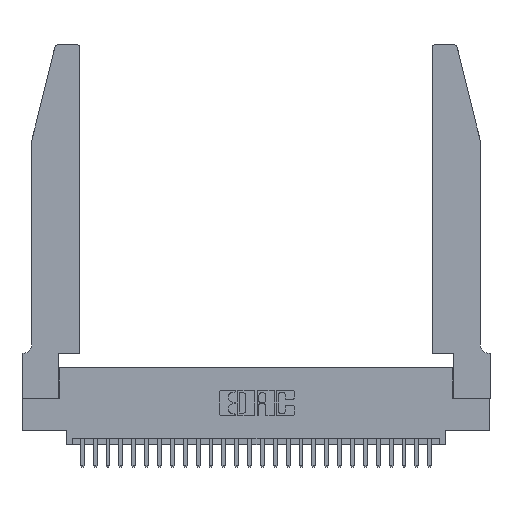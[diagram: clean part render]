
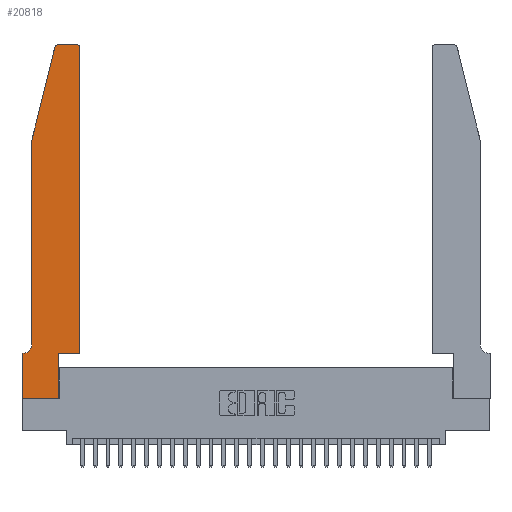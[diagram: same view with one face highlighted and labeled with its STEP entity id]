
A CAD part, top view. The second image highlights one B-rep face of the part: STEP entity #20818.
In plain terms, the highlighted planar face has unit normal (0, 0, 1).
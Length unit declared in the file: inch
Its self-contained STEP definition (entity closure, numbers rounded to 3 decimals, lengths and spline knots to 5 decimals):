
#77 = ORIENTED_EDGE ( 'NONE', *, *, #12620, .T. ) ;
#313 = LINE ( 'NONE', #23612, #17528 ) ;
#765 = VECTOR ( 'NONE', #23305, 39.37008 ) ;
#925 = ORIENTED_EDGE ( 'NONE', *, *, #25373, .T. ) ;
#2102 = ORIENTED_EDGE ( 'NONE', *, *, #21250, .T. ) ;
#2154 = CIRCLE ( 'NONE', #4100, 0.03 ) ;
#2333 = CARTESIAN_POINT ( 'NONE',  ( 0., 0., 0.37 ) ) ;
#2403 = CARTESIAN_POINT ( 'NONE',  ( 0.4505, 0.35, 0.37 ) ) ;
#2539 = LINE ( 'NONE', #8408, #19004 ) ;
#3184 = CARTESIAN_POINT ( 'NONE',  ( 0.0755, 0.35, 0.37 ) ) ;
#3295 = LINE ( 'NONE', #2333, #15235 ) ;
#3737 = LINE ( 'NONE', #22933, #20849 ) ;
#4062 = ORIENTED_EDGE ( 'NONE', *, *, #21682, .T. ) ;
#4100 = AXIS2_PLACEMENT_3D ( 'NONE', #22293, #8950, #24520 ) ;
#5616 = CARTESIAN_POINT ( 'NONE',  ( 0.0755, 2., 0.37 ) ) ;
#5730 = CARTESIAN_POINT ( 'NONE',  ( 0.25487, 2.72718, 0.37 ) ) ;
#5871 = VECTOR ( 'NONE', #13634, 39.37008 ) ;
#6180 = LINE ( 'NONE', #24738, #5871 ) ;
#6347 = VERTEX_POINT ( 'NONE', #12499 ) ;
#6475 = PLANE ( 'NONE',  #11710 ) ;
#6580 = ORIENTED_EDGE ( 'NONE', *, *, #26345, .T. ) ;
#6736 = EDGE_LOOP ( 'NONE', ( #25363, #77, #2102, #21582, #11714, #18321, #925, #13669, #13205, #16756, #4062, #6580 ) ) ;
#6796 = LINE ( 'NONE', #3184, #765 ) ;
#6835 = VERTEX_POINT ( 'NONE', #19029 ) ;
#7373 = CARTESIAN_POINT ( 'NONE',  ( 0.0055, 0.42, 0.37 ) ) ;
#7745 = LINE ( 'NONE', #8563, #12960 ) ;
#7884 = DIRECTION ( 'NONE',  ( 0., -1., 0. ) ) ;
#8408 = CARTESIAN_POINT ( 'NONE',  ( 0.2605, 2.75, 0.37 ) ) ;
#8563 = CARTESIAN_POINT ( 'NONE',  ( 0.2865, 0.35, 0.37 ) ) ;
#8651 = CARTESIAN_POINT ( 'NONE',  ( 0., 0.35, 0.37 ) ) ;
#8742 = DIRECTION ( 'NONE',  ( 0., 0., 1. ) ) ;
#8790 = EDGE_CURVE ( 'NONE', #16522, #6347, #6796, .T. ) ;
#8950 = DIRECTION ( 'NONE',  ( 0., 0., 1. ) ) ;
#8978 = EDGE_CURVE ( 'NONE', #26925, #25422, #2539, .T. ) ;
#9606 = DIRECTION ( 'NONE',  ( -1., 0., 0. ) ) ;
#11160 = DIRECTION ( 'NONE',  ( 0., -1., 0. ) ) ;
#11239 = CARTESIAN_POINT ( 'NONE',  ( 0.0055, 0.35, 0.37 ) ) ;
#11264 = CARTESIAN_POINT ( 'NONE',  ( 0.0755, 0.42, 0.37 ) ) ;
#11443 = CARTESIAN_POINT ( 'NONE',  ( 0.284, 2.75, 0.37 ) ) ;
#11710 = AXIS2_PLACEMENT_3D ( 'NONE', #8651, #8742, #24304 ) ;
#11714 = ORIENTED_EDGE ( 'NONE', *, *, #23083, .T. ) ;
#12499 = CARTESIAN_POINT ( 'NONE',  ( 0., 0.35, 0.37 ) ) ;
#12620 = EDGE_CURVE ( 'NONE', #25422, #22592, #2154, .T. ) ;
#12876 = DIRECTION ( 'NONE',  ( 0., 0., 1. ) ) ;
#12960 = VECTOR ( 'NONE', #23836, 39.37008 ) ;
#13051 = CIRCLE ( 'NONE', #24053, 0.03 ) ;
#13205 = ORIENTED_EDGE ( 'NONE', *, *, #13803, .T. ) ;
#13634 = DIRECTION ( 'NONE',  ( 0., 1., 0. ) ) ;
#13669 = ORIENTED_EDGE ( 'NONE', *, *, #27585, .T. ) ;
#13689 = EDGE_CURVE ( 'NONE', #22673, #27228, #28235, .T. ) ;
#13803 = EDGE_CURVE ( 'NONE', #6835, #14386, #7745, .T. ) ;
#14370 = AXIS2_PLACEMENT_3D ( 'NONE', #7373, #22957, #9606 ) ;
#14386 = VERTEX_POINT ( 'NONE', #21577 ) ;
#15052 = CARTESIAN_POINT ( 'NONE',  ( 0.4505, 2.72, 0.37 ) ) ;
#15235 = VECTOR ( 'NONE', #11160, 39.37008 ) ;
#15770 = VECTOR ( 'NONE', #7884, 39.37008 ) ;
#16522 = VERTEX_POINT ( 'NONE', #11239 ) ;
#16533 = CARTESIAN_POINT ( 'NONE',  ( 0.0755, 2., 0.37 ) ) ;
#16722 = DIRECTION ( 'NONE',  ( -0.239, -0.971, 0. ) ) ;
#16756 = ORIENTED_EDGE ( 'NONE', *, *, #21107, .T. ) ;
#17385 = VERTEX_POINT ( 'NONE', #20840 ) ;
#17390 = VECTOR ( 'NONE', #16722, 39.37008 ) ;
#17528 = VECTOR ( 'NONE', #25749, 39.37008 ) ;
#18321 = ORIENTED_EDGE ( 'NONE', *, *, #8790, .T. ) ;
#19004 = VECTOR ( 'NONE', #21754, 39.37008 ) ;
#19029 = CARTESIAN_POINT ( 'NONE',  ( 0.2865, 0., 0.37 ) ) ;
#19201 = CARTESIAN_POINT ( 'NONE',  ( 0.4205, 2.75, 0.37 ) ) ;
#20818 = ADVANCED_FACE ( 'NONE', ( #27769 ), #6475, .T. ) ;
#20840 = CARTESIAN_POINT ( 'NONE',  ( 0., 0., 0.37 ) ) ;
#20849 = VECTOR ( 'NONE', #25159, 39.37008 ) ;
#21107 = EDGE_CURVE ( 'NONE', #14386, #23605, #3737, .T. ) ;
#21250 = EDGE_CURVE ( 'NONE', #22592, #22673, #23288, .T. ) ;
#21433 = VERTEX_POINT ( 'NONE', #15052 ) ;
#21577 = CARTESIAN_POINT ( 'NONE',  ( 0.2865, 0.35, 0.37 ) ) ;
#21582 = ORIENTED_EDGE ( 'NONE', *, *, #13689, .T. ) ;
#21682 = EDGE_CURVE ( 'NONE', #23605, #21433, #6180, .T. ) ;
#21754 = DIRECTION ( 'NONE',  ( -1., 0., 0. ) ) ;
#22293 = CARTESIAN_POINT ( 'NONE',  ( 0.284, 2.72, 0.37 ) ) ;
#22592 = VERTEX_POINT ( 'NONE', #5730 ) ;
#22673 = VERTEX_POINT ( 'NONE', #25974 ) ;
#22933 = CARTESIAN_POINT ( 'NONE',  ( 0.4505, 0.35, 0.37 ) ) ;
#22957 = DIRECTION ( 'NONE',  ( 0., 0., -1. ) ) ;
#23083 = EDGE_CURVE ( 'NONE', #27228, #16522, #24261, .T. ) ;
#23288 = LINE ( 'NONE', #16533, #17390 ) ;
#23305 = DIRECTION ( 'NONE',  ( -1., 0., 0. ) ) ;
#23605 = VERTEX_POINT ( 'NONE', #2403 ) ;
#23612 = CARTESIAN_POINT ( 'NONE',  ( 0., 0., 0.37 ) ) ;
#23836 = DIRECTION ( 'NONE',  ( 0., 1., 0. ) ) ;
#24053 = AXIS2_PLACEMENT_3D ( 'NONE', #26198, #12876, #28384 ) ;
#24261 = CIRCLE ( 'NONE', #14370, 0.07 ) ;
#24304 = DIRECTION ( 'NONE',  ( 1., 0., 0. ) ) ;
#24520 = DIRECTION ( 'NONE',  ( 1., 0., 0. ) ) ;
#24738 = CARTESIAN_POINT ( 'NONE',  ( 0.4505, 0.35, 0.37 ) ) ;
#25159 = DIRECTION ( 'NONE',  ( 1., 0., 0. ) ) ;
#25363 = ORIENTED_EDGE ( 'NONE', *, *, #8978, .T. ) ;
#25373 = EDGE_CURVE ( 'NONE', #6347, #17385, #3295, .T. ) ;
#25422 = VERTEX_POINT ( 'NONE', #11443 ) ;
#25749 = DIRECTION ( 'NONE',  ( 1., 0., 0. ) ) ;
#25974 = CARTESIAN_POINT ( 'NONE',  ( 0.0755, 2., 0.37 ) ) ;
#26198 = CARTESIAN_POINT ( 'NONE',  ( 0.4205, 2.72, 0.37 ) ) ;
#26345 = EDGE_CURVE ( 'NONE', #21433, #26925, #13051, .T. ) ;
#26925 = VERTEX_POINT ( 'NONE', #19201 ) ;
#27228 = VERTEX_POINT ( 'NONE', #11264 ) ;
#27585 = EDGE_CURVE ( 'NONE', #17385, #6835, #313, .T. ) ;
#27769 = FACE_OUTER_BOUND ( 'NONE', #6736, .T. ) ;
#28235 = LINE ( 'NONE', #5616, #15770 ) ;
#28384 = DIRECTION ( 'NONE',  ( 1., 0., 0. ) ) ;
